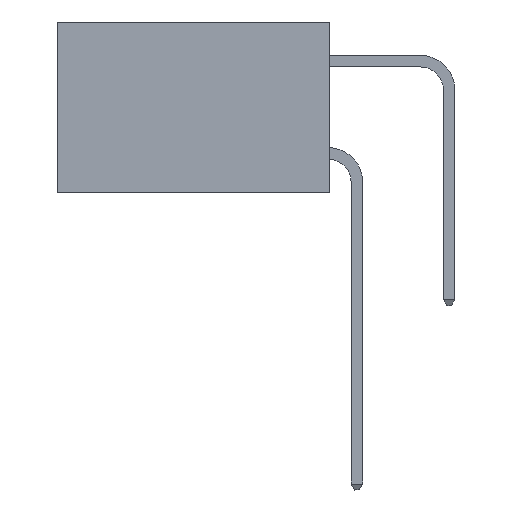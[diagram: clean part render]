
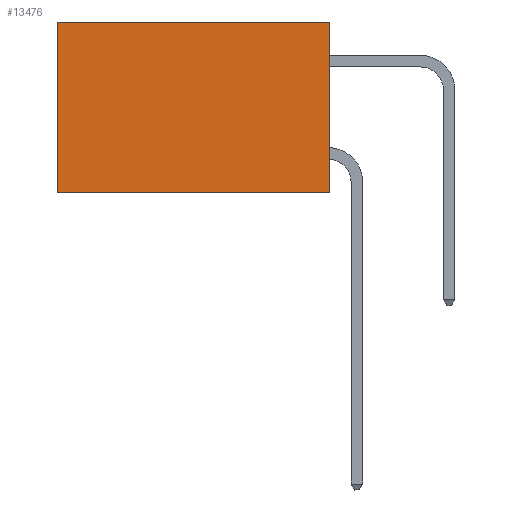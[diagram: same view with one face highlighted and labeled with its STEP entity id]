
A CAD part, left-side view. The second image highlights one B-rep face of the part: STEP entity #13476.
In plain terms, the highlighted planar face has unit normal (-1, 0, 0).
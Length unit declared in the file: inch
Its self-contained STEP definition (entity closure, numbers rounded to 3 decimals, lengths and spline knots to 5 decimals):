
#465 = ORIENTED_EDGE ( 'NONE', *, *, #6517, .F. ) ;
#828 = ORIENTED_EDGE ( 'NONE', *, *, #2139, .T. ) ;
#1910 = CARTESIAN_POINT ( 'NONE',  ( 0.277, 0., -0.37 ) ) ;
#2139 = EDGE_CURVE ( 'NONE', #14243, #2501, #10575, .T. ) ;
#2213 = CARTESIAN_POINT ( 'NONE',  ( 0.277, 0., 0. ) ) ;
#2501 = VERTEX_POINT ( 'NONE', #7002 ) ;
#3015 = VECTOR ( 'NONE', #22958, 39.37008 ) ;
#3626 = LINE ( 'NONE', #23190, #3015 ) ;
#3847 = DIRECTION ( 'NONE',  ( 0., 0., -1. ) ) ;
#4816 = EDGE_LOOP ( 'NONE', ( #10560, #12100, #465, #828 ) ) ;
#4999 = VECTOR ( 'NONE', #18156, 39.37008 ) ;
#6077 = EDGE_CURVE ( 'NONE', #2501, #15401, #3626, .T. ) ;
#6517 = EDGE_CURVE ( 'NONE', #14243, #18565, #10203, .T. ) ;
#6874 = LINE ( 'NONE', #23039, #20468 ) ;
#6978 = FACE_OUTER_BOUND ( 'NONE', #4816, .T. ) ;
#7002 = CARTESIAN_POINT ( 'NONE',  ( 0.277, 0.59, 0. ) ) ;
#10203 = LINE ( 'NONE', #18342, #4999 ) ;
#10560 = ORIENTED_EDGE ( 'NONE', *, *, #6077, .T. ) ;
#10575 = LINE ( 'NONE', #11710, #24540 ) ;
#11613 = PLANE ( 'NONE',  #15054 ) ;
#11710 = CARTESIAN_POINT ( 'NONE',  ( 0.277, 0., 0. ) ) ;
#12100 = ORIENTED_EDGE ( 'NONE', *, *, #15395, .F. ) ;
#13476 = ADVANCED_FACE ( 'NONE', ( #6978 ), #11613, .F. ) ;
#13589 = CARTESIAN_POINT ( 'NONE',  ( 0.277, 0.59, -0.37 ) ) ;
#14243 = VERTEX_POINT ( 'NONE', #2213 ) ;
#15054 = AXIS2_PLACEMENT_3D ( 'NONE', #1910, #15531, #3847 ) ;
#15395 = EDGE_CURVE ( 'NONE', #18565, #15401, #6874, .T. ) ;
#15401 = VERTEX_POINT ( 'NONE', #13589 ) ;
#15531 = DIRECTION ( 'NONE',  ( 1., 0., 0. ) ) ;
#18156 = DIRECTION ( 'NONE',  ( 0., 0., -1. ) ) ;
#18342 = CARTESIAN_POINT ( 'NONE',  ( 0.277, 0., -0.37 ) ) ;
#18565 = VERTEX_POINT ( 'NONE', #20488 ) ;
#19295 = DIRECTION ( 'NONE',  ( 0., 1., 0. ) ) ;
#20468 = VECTOR ( 'NONE', #19295, 39.37008 ) ;
#20488 = CARTESIAN_POINT ( 'NONE',  ( 0.277, 0., -0.37 ) ) ;
#22159 = DIRECTION ( 'NONE',  ( 0., 1., 0. ) ) ;
#22958 = DIRECTION ( 'NONE',  ( 0., 0., -1. ) ) ;
#23039 = CARTESIAN_POINT ( 'NONE',  ( 0.277, 0., -0.37 ) ) ;
#23190 = CARTESIAN_POINT ( 'NONE',  ( 0.277, 0.59, -0.37 ) ) ;
#24540 = VECTOR ( 'NONE', #22159, 39.37008 ) ;
